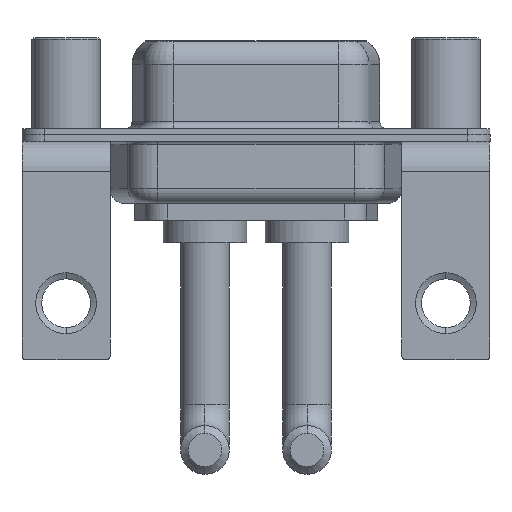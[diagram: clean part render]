
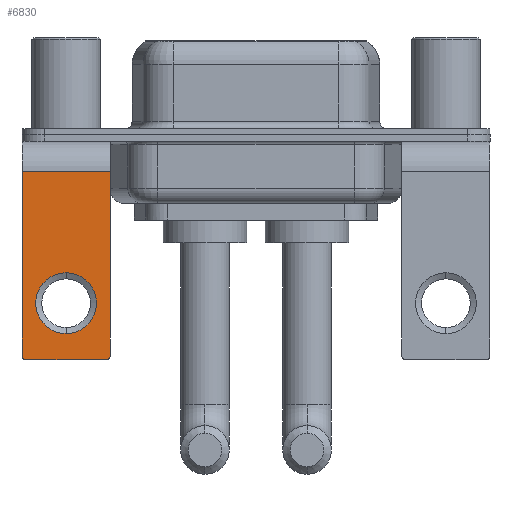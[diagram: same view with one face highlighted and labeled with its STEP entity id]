
A CAD part, front view. The second image highlights one B-rep face of the part: STEP entity #6830.
In plain terms, the highlighted planar face has unit normal (0, -1, 0).
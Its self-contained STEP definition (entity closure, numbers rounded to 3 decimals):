
#25 = CARTESIAN_POINT ( 'NONE',  ( -2.65, -6.25, -14.8 ) ) ;
#151 = CARTESIAN_POINT ( 'NONE',  ( 2.9, -6.25, -2.4 ) ) ;
#555 = CARTESIAN_POINT ( 'NONE',  ( 0., -6.25, -11.07 ) ) ;
#871 = EDGE_CURVE ( 'NONE', #11968, #2151, #5386, .T. ) ;
#1547 = ORIENTED_EDGE ( 'NONE', *, *, #1661, .T. ) ;
#1661 = EDGE_CURVE ( 'NONE', #8225, #9638, #2194, .T. ) ;
#1917 = VECTOR ( 'NONE', #3602, 1000. ) ;
#1993 = CIRCLE ( 'NONE', #14350, 0.25 ) ;
#2151 = VERTEX_POINT ( 'NONE', #25 ) ;
#2194 = CIRCLE ( 'NONE', #11206, 2. ) ;
#2902 = DIRECTION ( 'NONE',  ( 0., 0., 1. ) ) ;
#3141 = DIRECTION ( 'NONE',  ( -1., 0., 0. ) ) ;
#3154 = VERTEX_POINT ( 'NONE', #14464 ) ;
#3602 = DIRECTION ( 'NONE',  ( 0., 0., -1. ) ) ;
#3879 = ORIENTED_EDGE ( 'NONE', *, *, #4534, .T. ) ;
#3962 = DIRECTION ( 'NONE',  ( 0., 0., 1. ) ) ;
#4011 = CARTESIAN_POINT ( 'NONE',  ( 0., -6.25, -11.07 ) ) ;
#4018 = CARTESIAN_POINT ( 'NONE',  ( 0., -6.25, -13.07 ) ) ;
#4097 = AXIS2_PLACEMENT_3D ( 'NONE', #555, #10587, #3962 ) ;
#4158 = AXIS2_PLACEMENT_3D ( 'NONE', #151, #11162, #4677 ) ;
#4365 = EDGE_LOOP ( 'NONE', ( #1547, #10154 ) ) ;
#4417 = DIRECTION ( 'NONE',  ( -1., 0., 0. ) ) ;
#4534 = EDGE_CURVE ( 'NONE', #5935, #9274, #9245, .T. ) ;
#4677 = DIRECTION ( 'NONE',  ( 0., 0., 1. ) ) ;
#4770 = EDGE_CURVE ( 'NONE', #11968, #6172, #1993, .T. ) ;
#5119 = AXIS2_PLACEMENT_3D ( 'NONE', #12168, #10147, #14676 ) ;
#5386 = LINE ( 'NONE', #13340, #7711 ) ;
#5435 = VECTOR ( 'NONE', #10031, 1000. ) ;
#5513 = FACE_BOUND ( 'NONE', #4365, .T. ) ;
#5886 = VECTOR ( 'NONE', #3141, 1000. ) ;
#5935 = VERTEX_POINT ( 'NONE', #9480 ) ;
#6172 = VERTEX_POINT ( 'NONE', #13338 ) ;
#6352 = CARTESIAN_POINT ( 'NONE',  ( 2.65, -6.25, -14.55 ) ) ;
#6552 = LINE ( 'NONE', #6693, #5435 ) ;
#6693 = CARTESIAN_POINT ( 'NONE',  ( 2.9, -6.25, -2.4 ) ) ;
#6830 = ADVANCED_FACE ( 'NONE', ( #5513, #10333 ), #13747, .F. ) ;
#7023 = CARTESIAN_POINT ( 'NONE',  ( 0., -6.25, -9.07 ) ) ;
#7087 = EDGE_CURVE ( 'NONE', #9274, #2151, #9384, .T. ) ;
#7711 = VECTOR ( 'NONE', #4417, 1000. ) ;
#8225 = VERTEX_POINT ( 'NONE', #4018 ) ;
#8310 = EDGE_CURVE ( 'NONE', #3154, #6172, #6552, .T. ) ;
#8339 = ORIENTED_EDGE ( 'NONE', *, *, #871, .F. ) ;
#8376 = ORIENTED_EDGE ( 'NONE', *, *, #7087, .T. ) ;
#8925 = ORIENTED_EDGE ( 'NONE', *, *, #8310, .F. ) ;
#9000 = LINE ( 'NONE', #11021, #5886 ) ;
#9245 = LINE ( 'NONE', #13782, #1917 ) ;
#9274 = VERTEX_POINT ( 'NONE', #14548 ) ;
#9293 = CARTESIAN_POINT ( 'NONE',  ( 2.65, -6.25, -14.8 ) ) ;
#9318 = CIRCLE ( 'NONE', #4097, 2. ) ;
#9384 = CIRCLE ( 'NONE', #5119, 0.25 ) ;
#9480 = CARTESIAN_POINT ( 'NONE',  ( -2.9, -6.25, -2.4 ) ) ;
#9638 = VERTEX_POINT ( 'NONE', #7023 ) ;
#10031 = DIRECTION ( 'NONE',  ( 0., 0., -1. ) ) ;
#10090 = ORIENTED_EDGE ( 'NONE', *, *, #10501, .T. ) ;
#10147 = DIRECTION ( 'NONE',  ( 0., -1., 0. ) ) ;
#10154 = ORIENTED_EDGE ( 'NONE', *, *, #14016, .T. ) ;
#10333 = FACE_OUTER_BOUND ( 'NONE', #12289, .T. ) ;
#10501 = EDGE_CURVE ( 'NONE', #3154, #5935, #9000, .T. ) ;
#10587 = DIRECTION ( 'NONE',  ( 0., 1., 0. ) ) ;
#11021 = CARTESIAN_POINT ( 'NONE',  ( 2.9, -6.25, -2.4 ) ) ;
#11162 = DIRECTION ( 'NONE',  ( 0., 1., 0. ) ) ;
#11206 = AXIS2_PLACEMENT_3D ( 'NONE', #4011, #11827, #2902 ) ;
#11827 = DIRECTION ( 'NONE',  ( 0., 1., 0. ) ) ;
#11968 = VERTEX_POINT ( 'NONE', #9293 ) ;
#12073 = DIRECTION ( 'NONE',  ( 0., 0., 1. ) ) ;
#12168 = CARTESIAN_POINT ( 'NONE',  ( -2.65, -6.25, -14.55 ) ) ;
#12289 = EDGE_LOOP ( 'NONE', ( #3879, #8376, #8339, #14546, #8925, #10090 ) ) ;
#12349 = DIRECTION ( 'NONE',  ( 0., -1., 0. ) ) ;
#13338 = CARTESIAN_POINT ( 'NONE',  ( 2.9, -6.25, -14.55 ) ) ;
#13340 = CARTESIAN_POINT ( 'NONE',  ( 2.9, -6.25, -14.8 ) ) ;
#13747 = PLANE ( 'NONE',  #4158 ) ;
#13782 = CARTESIAN_POINT ( 'NONE',  ( -2.9, -6.25, -2.4 ) ) ;
#14016 = EDGE_CURVE ( 'NONE', #9638, #8225, #9318, .T. ) ;
#14350 = AXIS2_PLACEMENT_3D ( 'NONE', #6352, #12349, #12073 ) ;
#14464 = CARTESIAN_POINT ( 'NONE',  ( 2.9, -6.25, -2.4 ) ) ;
#14546 = ORIENTED_EDGE ( 'NONE', *, *, #4770, .T. ) ;
#14548 = CARTESIAN_POINT ( 'NONE',  ( -2.9, -6.25, -14.55 ) ) ;
#14676 = DIRECTION ( 'NONE',  ( 0., 0., 1. ) ) ;
